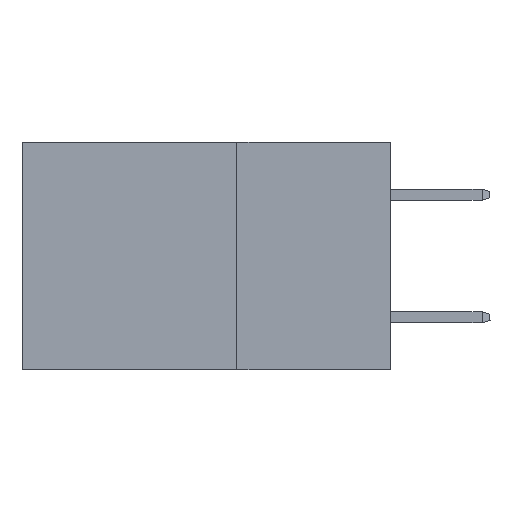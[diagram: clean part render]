
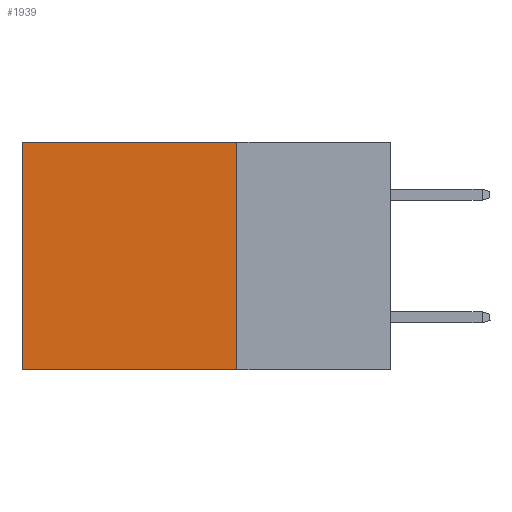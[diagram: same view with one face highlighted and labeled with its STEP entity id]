
A CAD part, left-side view. The second image highlights one B-rep face of the part: STEP entity #1939.
In plain terms, the highlighted planar face has unit normal (-1, 0, 0).
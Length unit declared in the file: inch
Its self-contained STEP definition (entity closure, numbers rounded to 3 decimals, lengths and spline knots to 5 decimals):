
#6 = EDGE_CURVE ( 'NONE', #13838, #14504, #27248, .T. ) ;
#1345 = FACE_OUTER_BOUND ( 'NONE', #15719, .T. ) ;
#1609 = LINE ( 'NONE', #20319, #17671 ) ;
#1939 = ADVANCED_FACE ( 'NONE', ( #1345 ), #17926, .F. ) ;
#2372 = VERTEX_POINT ( 'NONE', #25023 ) ;
#3080 = CARTESIAN_POINT ( 'NONE',  ( 0.2875, 0.6, 0. ) ) ;
#3404 = CARTESIAN_POINT ( 'NONE',  ( 0.2875, 0.25, -0.37 ) ) ;
#3735 = CARTESIAN_POINT ( 'NONE',  ( 0.2875, 0.25, 0. ) ) ;
#4219 = ORIENTED_EDGE ( 'NONE', *, *, #6, .F. ) ;
#4259 = AXIS2_PLACEMENT_3D ( 'NONE', #6275, #25854, #26066 ) ;
#4347 = VECTOR ( 'NONE', #29594, 39.37008 ) ;
#5526 = LINE ( 'NONE', #16030, #12645 ) ;
#5854 = DIRECTION ( 'NONE',  ( 0., 0., -1. ) ) ;
#6275 = CARTESIAN_POINT ( 'NONE',  ( 0.2875, 0.25, 0. ) ) ;
#7060 = ORIENTED_EDGE ( 'NONE', *, *, #23491, .T. ) ;
#7317 = DIRECTION ( 'NONE',  ( 0., 1., 0. ) ) ;
#7618 = CARTESIAN_POINT ( 'NONE',  ( 0.2875, 0.25, -0.37 ) ) ;
#7835 = ORIENTED_EDGE ( 'NONE', *, *, #11390, .F. ) ;
#7891 = VERTEX_POINT ( 'NONE', #3080 ) ;
#10699 = LINE ( 'NONE', #3735, #4347 ) ;
#11390 = EDGE_CURVE ( 'NONE', #2372, #13838, #5526, .T. ) ;
#12645 = VECTOR ( 'NONE', #25304, 39.37008 ) ;
#13838 = VERTEX_POINT ( 'NONE', #3404 ) ;
#14504 = VERTEX_POINT ( 'NONE', #16633 ) ;
#15719 = EDGE_LOOP ( 'NONE', ( #7060, #4219, #7835, #21345 ) ) ;
#16030 = CARTESIAN_POINT ( 'NONE',  ( 0.2875, 0.25, 0. ) ) ;
#16633 = CARTESIAN_POINT ( 'NONE',  ( 0.2875, 0.6, -0.37 ) ) ;
#17671 = VECTOR ( 'NONE', #5854, 39.37008 ) ;
#17926 = PLANE ( 'NONE',  #4259 ) ;
#20319 = CARTESIAN_POINT ( 'NONE',  ( 0.2875, 0.6, 0. ) ) ;
#21345 = ORIENTED_EDGE ( 'NONE', *, *, #22997, .T. ) ;
#22997 = EDGE_CURVE ( 'NONE', #2372, #7891, #10699, .T. ) ;
#23491 = EDGE_CURVE ( 'NONE', #7891, #14504, #1609, .T. ) ;
#25023 = CARTESIAN_POINT ( 'NONE',  ( 0.2875, 0.25, 0. ) ) ;
#25304 = DIRECTION ( 'NONE',  ( 0., 0., -1. ) ) ;
#25854 = DIRECTION ( 'NONE',  ( 1., 0., 0. ) ) ;
#26066 = DIRECTION ( 'NONE',  ( 0., 0., -1. ) ) ;
#26487 = VECTOR ( 'NONE', #7317, 39.37008 ) ;
#27248 = LINE ( 'NONE', #7618, #26487 ) ;
#29594 = DIRECTION ( 'NONE',  ( 0., 1., 0. ) ) ;
